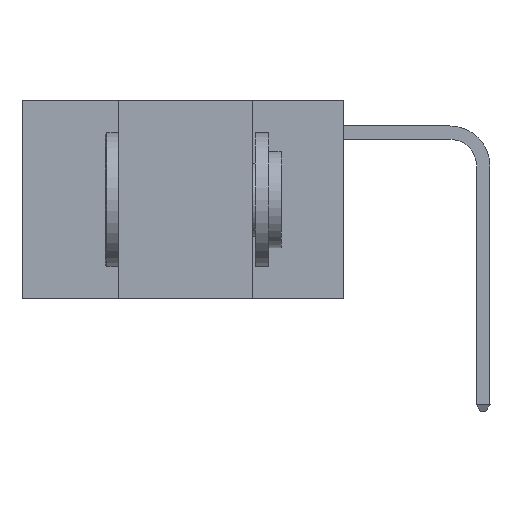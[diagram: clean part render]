
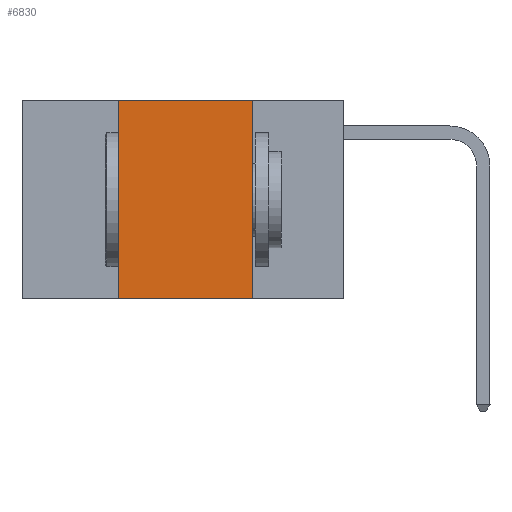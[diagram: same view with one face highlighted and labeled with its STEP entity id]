
A CAD part, left-side view. The second image highlights one B-rep face of the part: STEP entity #6830.
In plain terms, the highlighted planar face has unit normal (-1, 0, 0).
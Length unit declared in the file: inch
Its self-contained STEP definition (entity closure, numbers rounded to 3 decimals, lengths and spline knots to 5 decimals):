
#254 = DIRECTION ( 'NONE',  ( 0., 0., 1. ) ) ;
#275 = CARTESIAN_POINT ( 'NONE',  ( 0., 0.42, 0. ) ) ;
#547 = VECTOR ( 'NONE', #8238, 39.37008 ) ;
#714 = ORIENTED_EDGE ( 'NONE', *, *, #6730, .F. ) ;
#736 = LINE ( 'NONE', #4165, #779 ) ;
#779 = VECTOR ( 'NONE', #4205, 39.37008 ) ;
#878 = EDGE_CURVE ( 'NONE', #8260, #2920, #6051, .T. ) ;
#1078 = ORIENTED_EDGE ( 'NONE', *, *, #878, .F. ) ;
#1142 = EDGE_CURVE ( 'NONE', #2920, #8764, #7748, .T. ) ;
#1501 = ORIENTED_EDGE ( 'NONE', *, *, #7179, .T. ) ;
#2452 = FACE_OUTER_BOUND ( 'NONE', #7351, .T. ) ;
#2818 = AXIS2_PLACEMENT_3D ( 'NONE', #5838, #5712, #5245 ) ;
#2842 = LINE ( 'NONE', #275, #2944 ) ;
#2920 = VERTEX_POINT ( 'NONE', #5929 ) ;
#2944 = VECTOR ( 'NONE', #254, 39.37008 ) ;
#4165 = CARTESIAN_POINT ( 'NONE',  ( 0., 0.6, -0.37 ) ) ;
#4205 = DIRECTION ( 'NONE',  ( 0., -1., 0. ) ) ;
#5245 = DIRECTION ( 'NONE',  ( 0., 0., -1. ) ) ;
#5643 = CARTESIAN_POINT ( 'NONE',  ( 0., 0.17, -0.37 ) ) ;
#5712 = DIRECTION ( 'NONE',  ( 1., 0., 0. ) ) ;
#5838 = CARTESIAN_POINT ( 'NONE',  ( 0., 0.6, 0. ) ) ;
#5911 = VECTOR ( 'NONE', #9397, 39.37008 ) ;
#5929 = CARTESIAN_POINT ( 'NONE',  ( 0., 0.17, 0. ) ) ;
#6051 = LINE ( 'NONE', #8955, #5911 ) ;
#6614 = CARTESIAN_POINT ( 'NONE',  ( 0., 0.42, -0.37 ) ) ;
#6730 = EDGE_CURVE ( 'NONE', #9853, #8260, #2842, .T. ) ;
#6830 = ADVANCED_FACE ( 'NONE', ( #2452 ), #7267, .F. ) ;
#7179 = EDGE_CURVE ( 'NONE', #9853, #8764, #736, .T. ) ;
#7267 = PLANE ( 'NONE',  #2818 ) ;
#7351 = EDGE_LOOP ( 'NONE', ( #8707, #1078, #714, #1501 ) ) ;
#7748 = LINE ( 'NONE', #8448, #547 ) ;
#8238 = DIRECTION ( 'NONE',  ( 0., 0., -1. ) ) ;
#8260 = VERTEX_POINT ( 'NONE', #8624 ) ;
#8448 = CARTESIAN_POINT ( 'NONE',  ( 0., 0.17, 0. ) ) ;
#8624 = CARTESIAN_POINT ( 'NONE',  ( 0., 0.42, 0. ) ) ;
#8707 = ORIENTED_EDGE ( 'NONE', *, *, #1142, .F. ) ;
#8764 = VERTEX_POINT ( 'NONE', #5643 ) ;
#8955 = CARTESIAN_POINT ( 'NONE',  ( 0., 0.6, 0. ) ) ;
#9397 = DIRECTION ( 'NONE',  ( 0., -1., 0. ) ) ;
#9853 = VERTEX_POINT ( 'NONE', #6614 ) ;
